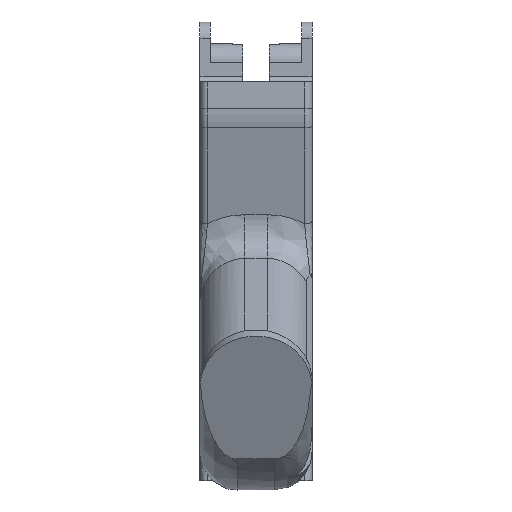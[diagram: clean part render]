
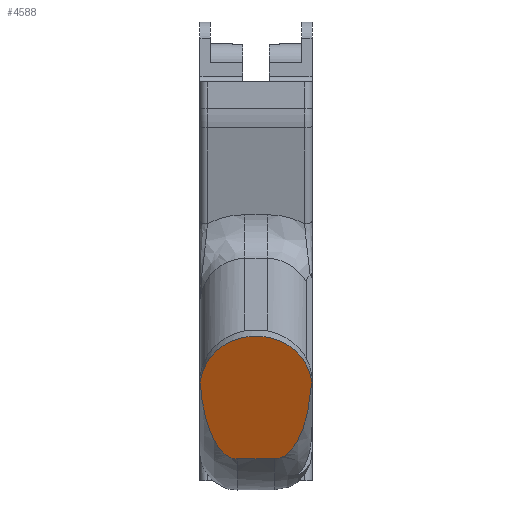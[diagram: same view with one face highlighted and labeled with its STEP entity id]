
A CAD part, front view. The second image highlights one B-rep face of the part: STEP entity #4588.
In plain terms, the highlighted planar face has unit normal (0, -0.913, -0.407).
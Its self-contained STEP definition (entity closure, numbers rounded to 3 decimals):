
#2993=CARTESIAN_POINT('',(-5.0,-97.487,-111.098));
#2994=VERTEX_POINT('',#2993);
#3024=CARTESIAN_POINT('',(-14.922,-106.649,-90.519));
#3025=VERTEX_POINT('',#3024);
#3026=CARTESIAN_POINT('',(-5.,-97.487,-111.098));
#3027=CARTESIAN_POINT('',(-5.52,-97.487,-111.098));
#3028=CARTESIAN_POINT('',(-6.023,-97.529,-111.003));
#3029=CARTESIAN_POINT('',(-7.114,-97.703,-110.612));
#3030=CARTESIAN_POINT('',(-7.668,-97.851,-110.279));
#3031=CARTESIAN_POINT('',(-9.001,-98.317,-109.234));
#3032=CARTESIAN_POINT('',(-9.712,-98.693,-108.388));
#3033=CARTESIAN_POINT('',(-11.401,-99.797,-105.909));
#3034=CARTESIAN_POINT('',(-12.358,-100.735,-103.801));
#3035=CARTESIAN_POINT('',(-14.099,-103.268,-98.113));
#3036=CARTESIAN_POINT('',(-14.715,-104.92,-94.403));
#3037=CARTESIAN_POINT('',(-14.922,-106.649,-90.519));
#3038=B_SPLINE_CURVE_WITH_KNOTS('',3,(#3026,#3027,#3028,#3029,#3030,#3031,#3032,#3033,#3034,#3035,#3036,#3037),.UNSPECIFIED.,.F.,.U.,(4,2,2,2,2,4),(0.0,0.156,0.351,0.682,1.307,2.114),.UNSPECIFIED.);
#3039=EDGE_CURVE('',#2994,#3025,#3038,.T.);
#3116=CARTESIAN_POINT('',(5.0,-97.487,-111.098));
#3117=VERTEX_POINT('',#3116);
#3146=CARTESIAN_POINT('',(0.0,-97.487,-111.098));
#3147=VERTEX_POINT('',#3146);
#3148=CARTESIAN_POINT('',(0.0,-97.487,-111.098));
#3149=DIRECTION('',(1.0,0.0,0.0));
#3150=VECTOR('',#3149,5.0);
#3151=LINE('',#3148,#3150);
#3152=EDGE_CURVE('',#3147,#3117,#3151,.T.);
#3154=CARTESIAN_POINT('',(0.0,-97.487,-111.098));
#3155=DIRECTION('',(-1.0,0.0,0.0));
#3156=VECTOR('',#3155,5.0);
#3157=LINE('',#3154,#3156);
#3158=EDGE_CURVE('',#3147,#2994,#3157,.T.);
#3388=CARTESIAN_POINT('',(14.922,-106.649,-90.519));
#3389=VERTEX_POINT('',#3388);
#3399=CARTESIAN_POINT('',(14.922,-106.649,-90.519));
#3400=CARTESIAN_POINT('',(14.654,-104.412,-95.544));
#3401=CARTESIAN_POINT('',(13.699,-102.311,-100.264));
#3402=CARTESIAN_POINT('',(11.255,-99.667,-106.2));
#3403=CARTESIAN_POINT('',(10.14,-98.867,-107.998));
#3404=CARTESIAN_POINT('',(8.358,-98.075,-109.778));
#3405=CARTESIAN_POINT('',(7.718,-97.851,-110.279));
#3406=CARTESIAN_POINT('',(6.68,-97.63,-110.776));
#3407=CARTESIAN_POINT('',(6.349,-97.576,-110.898));
#3408=CARTESIAN_POINT('',(5.674,-97.505,-111.057));
#3409=CARTESIAN_POINT('',(5.34,-97.487,-111.098));
#3410=CARTESIAN_POINT('',(5.,-97.487,-111.098));
#3411=B_SPLINE_CURVE_WITH_KNOTS('',3,(#3399,#3400,#3401,#3402,#3403,#3404,#3405,#3406,#3407,#3408,#3409,#3410),.UNSPECIFIED.,.F.,.U.,(4,2,2,2,2,4),(0.323,2.003,3.037,3.499,3.702,3.895),.UNSPECIFIED.);
#3412=EDGE_CURVE('',#3389,#3117,#3411,.T.);
#4560=CARTESIAN_POINT('',(0.0,-106.028,-91.914));
#4561=DIRECTION('',(0.,0.914,0.407));
#4562=DIRECTION('',(0.707,-0.288,0.646));
#4563=AXIS2_PLACEMENT_3D('',#4560,#4561,#4562);
#4564=CIRCLE('',#4563,15.);
#4565=EDGE_CURVE('',#3025,#3389,#4564,.T.);
#4576=CARTESIAN_POINT('',(0.0,-97.487,-111.098));
#4577=DIRECTION('',(0.0,-0.914,-0.407));
#4578=DIRECTION('',(0.0,0.407,-0.914));
#4579=AXIS2_PLACEMENT_3D('',#4576,#4577,#4578);
#4580=PLANE('',#4579);
#4581=ORIENTED_EDGE('',*,*,#3039,.F.);
#4582=ORIENTED_EDGE('',*,*,#3158,.F.);
#4583=ORIENTED_EDGE('',*,*,#3152,.T.);
#4584=ORIENTED_EDGE('',*,*,#3412,.F.);
#4585=ORIENTED_EDGE('',*,*,#4565,.F.);
#4586=EDGE_LOOP('',(#4581,#4582,#4583,#4584,#4585));
#4587=FACE_OUTER_BOUND('',#4586,.T.);
#4588=ADVANCED_FACE('',(#4587),#4580,.T.);
